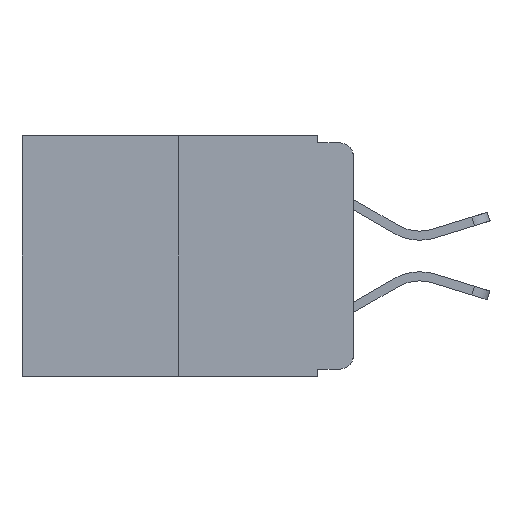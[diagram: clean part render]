
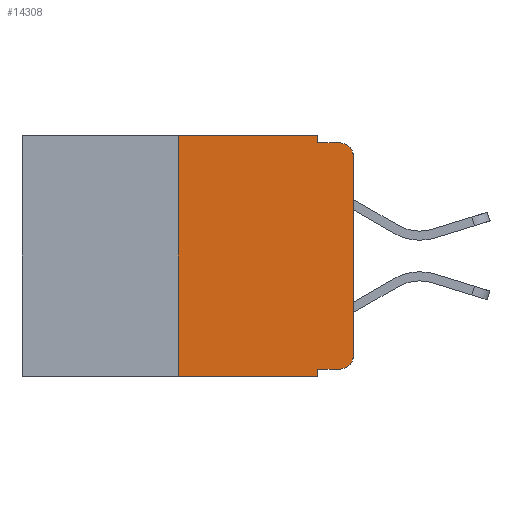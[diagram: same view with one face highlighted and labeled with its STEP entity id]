
A CAD part, left-side view. The second image highlights one B-rep face of the part: STEP entity #14308.
In plain terms, the highlighted planar face has unit normal (-1, 0, 0).
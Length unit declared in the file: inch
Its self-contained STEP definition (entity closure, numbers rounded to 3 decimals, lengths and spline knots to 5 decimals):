
#628 = DIRECTION ( 'NONE',  ( 0., 0., -1. ) ) ;
#977 = CARTESIAN_POINT ( 'NONE',  ( 0., 0.051, 0. ) ) ;
#982 = VECTOR ( 'NONE', #14587, 39.37008 ) ;
#1522 = VECTOR ( 'NONE', #11913, 39.37008 ) ;
#1623 = VECTOR ( 'NONE', #3257, 39.37008 ) ;
#1820 = DIRECTION ( 'NONE',  ( 0., -1., 0. ) ) ;
#1929 = CARTESIAN_POINT ( 'NONE',  ( 0., 0.473, 0. ) ) ;
#2284 = EDGE_CURVE ( 'NONE', #16206, #20858, #6460, .T. ) ;
#2366 = CARTESIAN_POINT ( 'NONE',  ( 0., 0., -0.313 ) ) ;
#2791 = VERTEX_POINT ( 'NONE', #13238 ) ;
#2934 = LINE ( 'NONE', #9630, #7863 ) ;
#3257 = DIRECTION ( 'NONE',  ( 0., -1., 0. ) ) ;
#4072 = VERTEX_POINT ( 'NONE', #18529 ) ;
#4682 = CARTESIAN_POINT ( 'NONE',  ( 0., 0.473, -0.343 ) ) ;
#5151 = VERTEX_POINT ( 'NONE', #16146 ) ;
#5835 = ORIENTED_EDGE ( 'NONE', *, *, #13781, .T. ) ;
#6040 = LINE ( 'NONE', #13416, #19203 ) ;
#6396 = VERTEX_POINT ( 'NONE', #19606 ) ;
#6460 = LINE ( 'NONE', #18451, #1522 ) ;
#6541 = CARTESIAN_POINT ( 'NONE',  ( 0., 0.02, -0.333 ) ) ;
#6719 = CIRCLE ( 'NONE', #21052, 0.02 ) ;
#6942 = DIRECTION ( 'NONE',  ( 0., 0., -1. ) ) ;
#7258 = VERTEX_POINT ( 'NONE', #18327 ) ;
#7863 = VECTOR ( 'NONE', #21041, 39.37008 ) ;
#7870 = VERTEX_POINT ( 'NONE', #10137 ) ;
#8069 = VECTOR ( 'NONE', #21082, 39.37008 ) ;
#8695 = FACE_OUTER_BOUND ( 'NONE', #11297, .T. ) ;
#8985 = ORIENTED_EDGE ( 'NONE', *, *, #14063, .T. ) ;
#9056 = CARTESIAN_POINT ( 'NONE',  ( 0., 0.25, 0. ) ) ;
#9451 = VERTEX_POINT ( 'NONE', #977 ) ;
#9493 = CARTESIAN_POINT ( 'NONE',  ( 0., 0.02, -0.03 ) ) ;
#9630 = CARTESIAN_POINT ( 'NONE',  ( 0., 0.051, 0. ) ) ;
#9820 = AXIS2_PLACEMENT_3D ( 'NONE', #9493, #20903, #11153 ) ;
#9842 = LINE ( 'NONE', #4682, #982 ) ;
#10137 = CARTESIAN_POINT ( 'NONE',  ( 0., 0.02, -0.01 ) ) ;
#10455 = VECTOR ( 'NONE', #11221, 39.37008 ) ;
#10541 = ORIENTED_EDGE ( 'NONE', *, *, #15972, .F. ) ;
#10570 = DIRECTION ( 'NONE',  ( -1., 0., 0. ) ) ;
#10724 = ORIENTED_EDGE ( 'NONE', *, *, #2284, .T. ) ;
#11153 = DIRECTION ( 'NONE',  ( 0., 0., -1. ) ) ;
#11188 = VECTOR ( 'NONE', #18906, 39.37008 ) ;
#11221 = DIRECTION ( 'NONE',  ( 0., 0., -1. ) ) ;
#11222 = ORIENTED_EDGE ( 'NONE', *, *, #18204, .F. ) ;
#11297 = EDGE_LOOP ( 'NONE', ( #10724, #13829, #15815, #11222, #11470, #19962, #8985, #10541, #19268, #5835 ) ) ;
#11346 = CARTESIAN_POINT ( 'NONE',  ( 0., 0.051, -0.01 ) ) ;
#11470 = ORIENTED_EDGE ( 'NONE', *, *, #20489, .F. ) ;
#11518 = CARTESIAN_POINT ( 'NONE',  ( 0., 0.473, 0. ) ) ;
#11913 = DIRECTION ( 'NONE',  ( 0., 0., 1. ) ) ;
#12546 = CARTESIAN_POINT ( 'NONE',  ( 0., 0., -0.03 ) ) ;
#13238 = CARTESIAN_POINT ( 'NONE',  ( 0., 0.051, -0.333 ) ) ;
#13416 = CARTESIAN_POINT ( 'NONE',  ( 0., 0.051, -0.333 ) ) ;
#13781 = EDGE_CURVE ( 'NONE', #19332, #16206, #6719, .T. ) ;
#13829 = ORIENTED_EDGE ( 'NONE', *, *, #20342, .T. ) ;
#14063 = EDGE_CURVE ( 'NONE', #5151, #6396, #9842, .T. ) ;
#14308 = ADVANCED_FACE ( 'NONE', ( #8695 ), #15074, .F. ) ;
#14437 = CARTESIAN_POINT ( 'NONE',  ( 0., 0.051, 0. ) ) ;
#14587 = DIRECTION ( 'NONE',  ( 0., -1., 0. ) ) ;
#14824 = LINE ( 'NONE', #11518, #1623 ) ;
#14830 = LINE ( 'NONE', #14437, #10455 ) ;
#14884 = EDGE_CURVE ( 'NONE', #2791, #19332, #6040, .T. ) ;
#15074 = PLANE ( 'NONE',  #18127 ) ;
#15815 = ORIENTED_EDGE ( 'NONE', *, *, #19267, .F. ) ;
#15972 = EDGE_CURVE ( 'NONE', #2791, #6396, #14830, .T. ) ;
#16057 = LINE ( 'NONE', #9056, #11188 ) ;
#16146 = CARTESIAN_POINT ( 'NONE',  ( 0., 0.25, -0.343 ) ) ;
#16206 = VERTEX_POINT ( 'NONE', #2366 ) ;
#16814 = DIRECTION ( 'NONE',  ( 1., 0., 0. ) ) ;
#17104 = EDGE_CURVE ( 'NONE', #5151, #7258, #16057, .T. ) ;
#17425 = CIRCLE ( 'NONE', #9820, 0.02 ) ;
#18127 = AXIS2_PLACEMENT_3D ( 'NONE', #1929, #16814, #6942 ) ;
#18204 = EDGE_CURVE ( 'NONE', #9451, #4072, #2934, .T. ) ;
#18327 = CARTESIAN_POINT ( 'NONE',  ( 0., 0.25, 0. ) ) ;
#18451 = CARTESIAN_POINT ( 'NONE',  ( 0., 0., 0. ) ) ;
#18529 = CARTESIAN_POINT ( 'NONE',  ( 0., 0.051, -0.01 ) ) ;
#18906 = DIRECTION ( 'NONE',  ( 0., 0., 1. ) ) ;
#19203 = VECTOR ( 'NONE', #1820, 39.37008 ) ;
#19267 = EDGE_CURVE ( 'NONE', #4072, #7870, #20618, .T. ) ;
#19268 = ORIENTED_EDGE ( 'NONE', *, *, #14884, .T. ) ;
#19332 = VERTEX_POINT ( 'NONE', #6541 ) ;
#19606 = CARTESIAN_POINT ( 'NONE',  ( 0., 0.051, -0.343 ) ) ;
#19962 = ORIENTED_EDGE ( 'NONE', *, *, #17104, .F. ) ;
#20342 = EDGE_CURVE ( 'NONE', #20858, #7870, #17425, .T. ) ;
#20372 = CARTESIAN_POINT ( 'NONE',  ( 0., 0.02, -0.313 ) ) ;
#20489 = EDGE_CURVE ( 'NONE', #7258, #9451, #14824, .T. ) ;
#20618 = LINE ( 'NONE', #11346, #8069 ) ;
#20858 = VERTEX_POINT ( 'NONE', #12546 ) ;
#20903 = DIRECTION ( 'NONE',  ( -1., 0., 0. ) ) ;
#21041 = DIRECTION ( 'NONE',  ( 0., 0., -1. ) ) ;
#21052 = AXIS2_PLACEMENT_3D ( 'NONE', #20372, #10570, #628 ) ;
#21082 = DIRECTION ( 'NONE',  ( 0., -1., 0. ) ) ;
